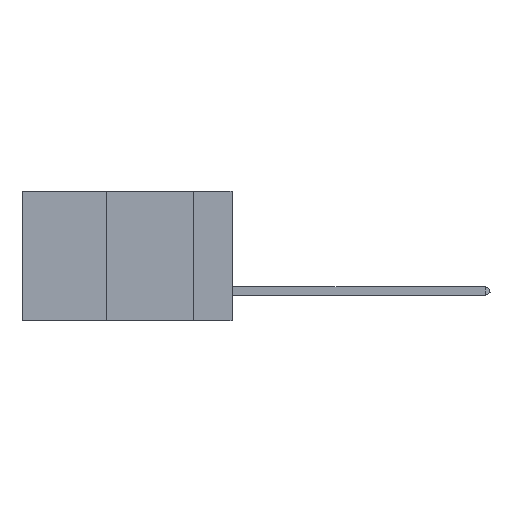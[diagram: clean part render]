
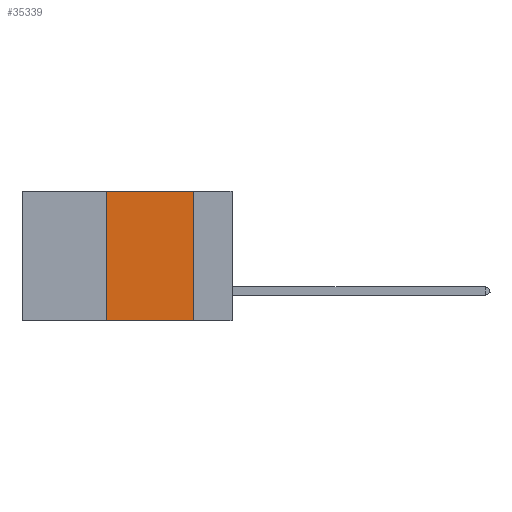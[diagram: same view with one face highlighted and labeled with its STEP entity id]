
A CAD part, left-side view. The second image highlights one B-rep face of the part: STEP entity #35339.
In plain terms, the highlighted planar face has unit normal (-1, 0, 0).
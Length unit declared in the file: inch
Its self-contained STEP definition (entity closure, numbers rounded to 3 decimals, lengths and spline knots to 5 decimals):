
#1346 = VECTOR ( 'NONE', #21772, 39.37008 ) ;
#2198 = CARTESIAN_POINT ( 'NONE',  ( 0., 0.36, 0. ) ) ;
#4029 = PLANE ( 'NONE',  #22897 ) ;
#5297 = VECTOR ( 'NONE', #21785, 39.37008 ) ;
#7473 = ORIENTED_EDGE ( 'NONE', *, *, #32731, .T. ) ;
#7821 = DIRECTION ( 'NONE',  ( 1., 0., 0. ) ) ;
#9296 = VECTOR ( 'NONE', #18075, 39.37008 ) ;
#11733 = LINE ( 'NONE', #2198, #27530 ) ;
#12051 = CARTESIAN_POINT ( 'NONE',  ( 0., 0.6, 0. ) ) ;
#12385 = VERTEX_POINT ( 'NONE', #25727 ) ;
#13273 = VERTEX_POINT ( 'NONE', #35949 ) ;
#13826 = EDGE_CURVE ( 'NONE', #30340, #12385, #11733, .T. ) ;
#14108 = ORIENTED_EDGE ( 'NONE', *, *, #41689, .F. ) ;
#15314 = CARTESIAN_POINT ( 'NONE',  ( 0., 0.6, -0.37 ) ) ;
#17770 = CARTESIAN_POINT ( 'NONE',  ( 0., 0.6, 0. ) ) ;
#18075 = DIRECTION ( 'NONE',  ( 0., -1., 0. ) ) ;
#18585 = LINE ( 'NONE', #35327, #1346 ) ;
#20402 = CARTESIAN_POINT ( 'NONE',  ( 0., 0.11, -0.37 ) ) ;
#21464 = EDGE_CURVE ( 'NONE', #13273, #30847, #18585, .T. ) ;
#21772 = DIRECTION ( 'NONE',  ( 0., 0., -1. ) ) ;
#21785 = DIRECTION ( 'NONE',  ( 0., -1., 0. ) ) ;
#22897 = AXIS2_PLACEMENT_3D ( 'NONE', #17770, #7821, #23722 ) ;
#23722 = DIRECTION ( 'NONE',  ( 0., 0., -1. ) ) ;
#24975 = LINE ( 'NONE', #12051, #5297 ) ;
#25727 = CARTESIAN_POINT ( 'NONE',  ( 0., 0.36, 0. ) ) ;
#27530 = VECTOR ( 'NONE', #34403, 39.37008 ) ;
#28226 = LINE ( 'NONE', #15314, #9296 ) ;
#28554 = ORIENTED_EDGE ( 'NONE', *, *, #21464, .F. ) ;
#30065 = ORIENTED_EDGE ( 'NONE', *, *, #13826, .F. ) ;
#30105 = CARTESIAN_POINT ( 'NONE',  ( 0., 0.36, -0.37 ) ) ;
#30340 = VERTEX_POINT ( 'NONE', #30105 ) ;
#30847 = VERTEX_POINT ( 'NONE', #20402 ) ;
#32731 = EDGE_CURVE ( 'NONE', #30340, #30847, #28226, .T. ) ;
#34403 = DIRECTION ( 'NONE',  ( 0., 0., 1. ) ) ;
#35327 = CARTESIAN_POINT ( 'NONE',  ( 0., 0.11, 0. ) ) ;
#35339 = ADVANCED_FACE ( 'NONE', ( #37053 ), #4029, .F. ) ;
#35949 = CARTESIAN_POINT ( 'NONE',  ( 0., 0.11, 0. ) ) ;
#37053 = FACE_OUTER_BOUND ( 'NONE', #41844, .T. ) ;
#41689 = EDGE_CURVE ( 'NONE', #12385, #13273, #24975, .T. ) ;
#41844 = EDGE_LOOP ( 'NONE', ( #28554, #14108, #30065, #7473 ) ) ;
